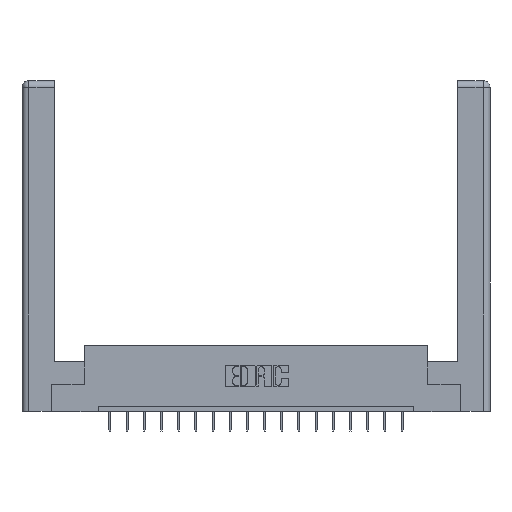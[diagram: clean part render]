
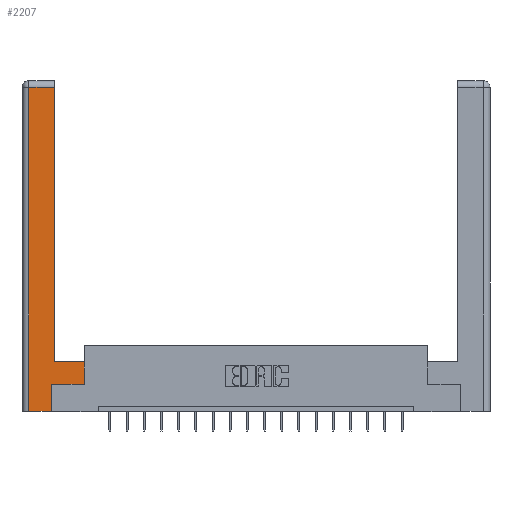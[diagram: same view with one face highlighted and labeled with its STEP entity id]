
A CAD part, top view. The second image highlights one B-rep face of the part: STEP entity #2207.
In plain terms, the highlighted planar face has unit normal (0, 0, 1).
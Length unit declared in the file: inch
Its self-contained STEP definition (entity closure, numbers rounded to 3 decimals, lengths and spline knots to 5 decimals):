
#288 = ORIENTED_EDGE ( 'NONE', *, *, #8654, .T. ) ;
#427 = LINE ( 'NONE', #10421, #10000 ) ;
#756 = VERTEX_POINT ( 'NONE', #12690 ) ;
#844 = ORIENTED_EDGE ( 'NONE', *, *, #5639, .T. ) ;
#963 = DIRECTION ( 'NONE',  ( 0., 1., 0. ) ) ;
#1333 = VECTOR ( 'NONE', #1817, 39.37008 ) ;
#1460 = LINE ( 'NONE', #15434, #3274 ) ;
#1514 = CARTESIAN_POINT ( 'NONE',  ( 0.565, 0.245, 0. ) ) ;
#1817 = DIRECTION ( 'NONE',  ( 0., -1., 0. ) ) ;
#1962 = DIRECTION ( 'NONE',  ( -1., 0., 0. ) ) ;
#2207 = ADVANCED_FACE ( 'NONE', ( #16982 ), #3220, .F. ) ;
#2424 = VERTEX_POINT ( 'NONE', #11613 ) ;
#2465 = EDGE_CURVE ( 'NONE', #4383, #2424, #18828, .T. ) ;
#2484 = VECTOR ( 'NONE', #18096, 39.37008 ) ;
#2894 = EDGE_CURVE ( 'NONE', #2424, #756, #14336, .T. ) ;
#3220 = PLANE ( 'NONE',  #16226 ) ;
#3274 = VECTOR ( 'NONE', #9707, 39.37008 ) ;
#3633 = CARTESIAN_POINT ( 'NONE',  ( 0.265, 0., 0. ) ) ;
#3808 = VERTEX_POINT ( 'NONE', #16629 ) ;
#4083 = CARTESIAN_POINT ( 'NONE',  ( 0.565, 0.45, 0. ) ) ;
#4383 = VERTEX_POINT ( 'NONE', #8627 ) ;
#4591 = LINE ( 'NONE', #5462, #16414 ) ;
#4648 = DIRECTION ( 'NONE',  ( -1., 0., 0. ) ) ;
#5419 = ORIENTED_EDGE ( 'NONE', *, *, #15446, .T. ) ;
#5462 = CARTESIAN_POINT ( 'NONE',  ( 0.265, 0., 0. ) ) ;
#5639 = EDGE_CURVE ( 'NONE', #16941, #4383, #7774, .T. ) ;
#6004 = VERTEX_POINT ( 'NONE', #12395 ) ;
#7383 = CARTESIAN_POINT ( 'NONE',  ( 0.0615, 2.94, 0. ) ) ;
#7731 = CARTESIAN_POINT ( 'NONE',  ( 0.565, 0.245, 0. ) ) ;
#7738 = DIRECTION ( 'NONE',  ( 0., 0., -1. ) ) ;
#7774 = LINE ( 'NONE', #13064, #17923 ) ;
#8627 = CARTESIAN_POINT ( 'NONE',  ( 0.295, 2.94, 0. ) ) ;
#8654 = EDGE_CURVE ( 'NONE', #3808, #16371, #9276, .T. ) ;
#9176 = EDGE_CURVE ( 'NONE', #6004, #16941, #427, .T. ) ;
#9276 = LINE ( 'NONE', #7731, #2484 ) ;
#9707 = DIRECTION ( 'NONE',  ( 0., 1., 0. ) ) ;
#9788 = EDGE_CURVE ( 'NONE', #756, #13962, #4591, .T. ) ;
#9937 = ORIENTED_EDGE ( 'NONE', *, *, #9788, .T. ) ;
#10000 = VECTOR ( 'NONE', #1962, 39.37008 ) ;
#10298 = LINE ( 'NONE', #4083, #16681 ) ;
#10421 = CARTESIAN_POINT ( 'NONE',  ( 0.295, 0.45, 0. ) ) ;
#10799 = VECTOR ( 'NONE', #18917, 39.37008 ) ;
#11613 = CARTESIAN_POINT ( 'NONE',  ( 0.0615, 2.94, 0. ) ) ;
#12395 = CARTESIAN_POINT ( 'NONE',  ( 0.565, 0.45, 0. ) ) ;
#12550 = ORIENTED_EDGE ( 'NONE', *, *, #2465, .T. ) ;
#12690 = CARTESIAN_POINT ( 'NONE',  ( 0.0615, 0., 0. ) ) ;
#12880 = ORIENTED_EDGE ( 'NONE', *, *, #2894, .T. ) ;
#13064 = CARTESIAN_POINT ( 'NONE',  ( 0.295, 3., 0. ) ) ;
#13840 = CARTESIAN_POINT ( 'NONE',  ( 0.295, 0.45, 0. ) ) ;
#13962 = VERTEX_POINT ( 'NONE', #3633 ) ;
#14336 = LINE ( 'NONE', #16601, #1333 ) ;
#15305 = EDGE_CURVE ( 'NONE', #13962, #3808, #1460, .T. ) ;
#15434 = CARTESIAN_POINT ( 'NONE',  ( 0.265, 0.245, 0. ) ) ;
#15446 = EDGE_CURVE ( 'NONE', #16371, #6004, #10298, .T. ) ;
#16226 = AXIS2_PLACEMENT_3D ( 'NONE', #16555, #7738, #4648 ) ;
#16371 = VERTEX_POINT ( 'NONE', #1514 ) ;
#16414 = VECTOR ( 'NONE', #17085, 39.37008 ) ;
#16456 = ORIENTED_EDGE ( 'NONE', *, *, #9176, .T. ) ;
#16555 = CARTESIAN_POINT ( 'NONE',  ( 0., 0., 0. ) ) ;
#16601 = CARTESIAN_POINT ( 'NONE',  ( 0.0615, 0., 0. ) ) ;
#16629 = CARTESIAN_POINT ( 'NONE',  ( 0.265, 0.245, 0. ) ) ;
#16681 = VECTOR ( 'NONE', #963, 39.37008 ) ;
#16941 = VERTEX_POINT ( 'NONE', #13840 ) ;
#16982 = FACE_OUTER_BOUND ( 'NONE', #19095, .T. ) ;
#17085 = DIRECTION ( 'NONE',  ( 1., 0., 0. ) ) ;
#17466 = ORIENTED_EDGE ( 'NONE', *, *, #15305, .T. ) ;
#17923 = VECTOR ( 'NONE', #18904, 39.37008 ) ;
#18096 = DIRECTION ( 'NONE',  ( 1., 0., 0. ) ) ;
#18828 = LINE ( 'NONE', #7383, #10799 ) ;
#18904 = DIRECTION ( 'NONE',  ( 0., 1., 0. ) ) ;
#18917 = DIRECTION ( 'NONE',  ( -1., 0., 0. ) ) ;
#19095 = EDGE_LOOP ( 'NONE', ( #844, #12550, #12880, #9937, #17466, #288, #5419, #16456 ) ) ;
